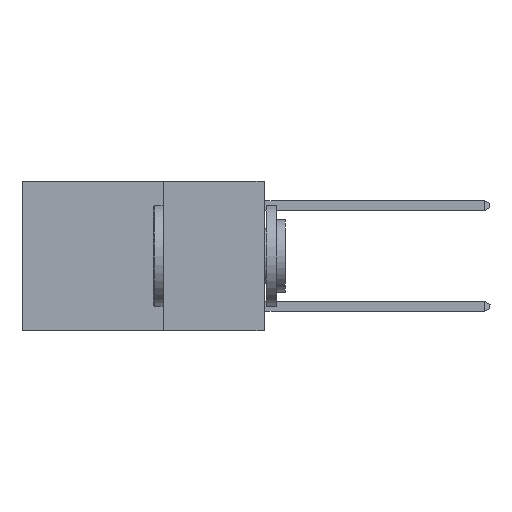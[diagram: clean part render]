
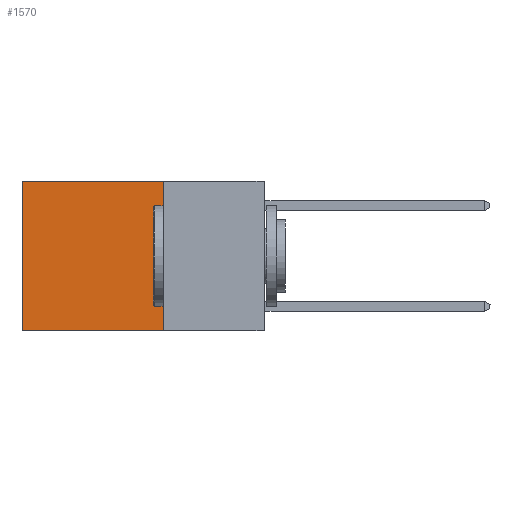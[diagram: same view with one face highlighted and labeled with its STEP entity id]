
A CAD part, left-side view. The second image highlights one B-rep face of the part: STEP entity #1570.
In plain terms, the highlighted planar face has unit normal (-1, 0, 0).
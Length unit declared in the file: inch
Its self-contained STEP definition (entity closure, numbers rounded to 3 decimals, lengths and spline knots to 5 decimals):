
#1090 = CARTESIAN_POINT ( 'NONE',  ( 0.2625, 0.6, 0. ) ) ;
#1570 = ADVANCED_FACE ( 'NONE', ( #3177 ), #10987, .F. ) ;
#1771 = VERTEX_POINT ( 'NONE', #6580 ) ;
#1975 = ORIENTED_EDGE ( 'NONE', *, *, #7950, .F. ) ;
#2449 = VECTOR ( 'NONE', #7270, 39.37008 ) ;
#2486 = CARTESIAN_POINT ( 'NONE',  ( 0.2625, 0.25, -0.37 ) ) ;
#3177 = FACE_OUTER_BOUND ( 'NONE', #10479, .T. ) ;
#3340 = EDGE_CURVE ( 'NONE', #9370, #6000, #10959, .T. ) ;
#3990 = AXIS2_PLACEMENT_3D ( 'NONE', #4437, #4498, #5694 ) ;
#4168 = CARTESIAN_POINT ( 'NONE',  ( 0.2625, 0.25, 0. ) ) ;
#4437 = CARTESIAN_POINT ( 'NONE',  ( 0.2625, 0.25, 0. ) ) ;
#4498 = DIRECTION ( 'NONE',  ( 1., 0., 0. ) ) ;
#4524 = DIRECTION ( 'NONE',  ( 0., 1., 0. ) ) ;
#5024 = CARTESIAN_POINT ( 'NONE',  ( 0.2625, 0.6, -0.37 ) ) ;
#5169 = EDGE_CURVE ( 'NONE', #1771, #13126, #7665, .T. ) ;
#5239 = DIRECTION ( 'NONE',  ( 0., 1., 0. ) ) ;
#5694 = DIRECTION ( 'NONE',  ( 0., 0., -1. ) ) ;
#6000 = VERTEX_POINT ( 'NONE', #2486 ) ;
#6580 = CARTESIAN_POINT ( 'NONE',  ( 0.2625, 0.6, 0. ) ) ;
#6851 = LINE ( 'NONE', #4168, #12065 ) ;
#6856 = ORIENTED_EDGE ( 'NONE', *, *, #3340, .F. ) ;
#7270 = DIRECTION ( 'NONE',  ( 0., 0., -1. ) ) ;
#7550 = DIRECTION ( 'NONE',  ( 0., 0., -1. ) ) ;
#7665 = LINE ( 'NONE', #1090, #12793 ) ;
#7950 = EDGE_CURVE ( 'NONE', #6000, #13126, #13351, .T. ) ;
#7958 = CARTESIAN_POINT ( 'NONE',  ( 0.2625, 0.25, 0. ) ) ;
#9370 = VERTEX_POINT ( 'NONE', #13547 ) ;
#9415 = ORIENTED_EDGE ( 'NONE', *, *, #5169, .T. ) ;
#10073 = VECTOR ( 'NONE', #4524, 39.37008 ) ;
#10106 = EDGE_CURVE ( 'NONE', #9370, #1771, #6851, .T. ) ;
#10479 = EDGE_LOOP ( 'NONE', ( #9415, #1975, #6856, #10569 ) ) ;
#10569 = ORIENTED_EDGE ( 'NONE', *, *, #10106, .T. ) ;
#10959 = LINE ( 'NONE', #7958, #2449 ) ;
#10987 = PLANE ( 'NONE',  #3990 ) ;
#11856 = CARTESIAN_POINT ( 'NONE',  ( 0.2625, 0.25, -0.37 ) ) ;
#12065 = VECTOR ( 'NONE', #5239, 39.37008 ) ;
#12793 = VECTOR ( 'NONE', #7550, 39.37008 ) ;
#13126 = VERTEX_POINT ( 'NONE', #5024 ) ;
#13351 = LINE ( 'NONE', #11856, #10073 ) ;
#13547 = CARTESIAN_POINT ( 'NONE',  ( 0.2625, 0.25, 0. ) ) ;
